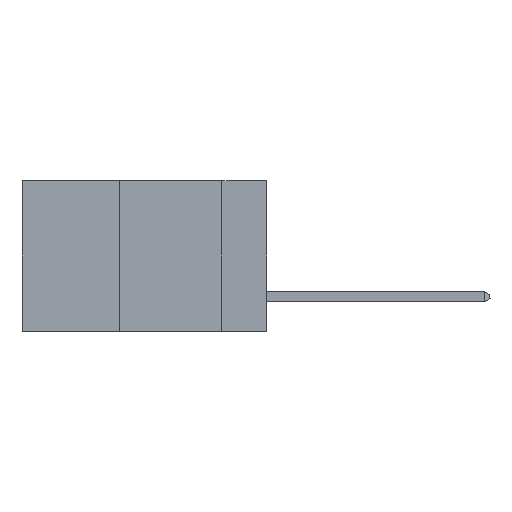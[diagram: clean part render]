
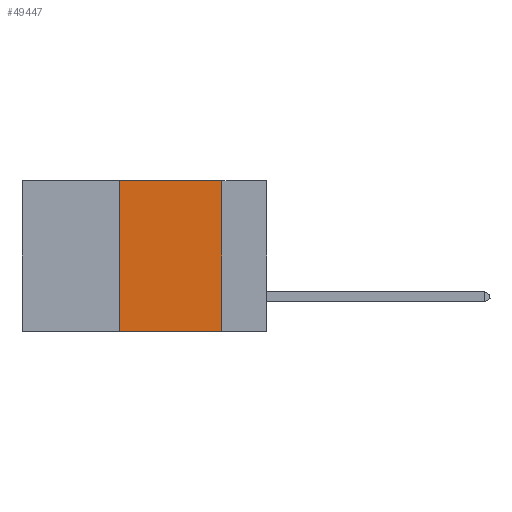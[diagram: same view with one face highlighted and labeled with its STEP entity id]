
A CAD part, left-side view. The second image highlights one B-rep face of the part: STEP entity #49447.
In plain terms, the highlighted planar face has unit normal (-1, 0, 0).
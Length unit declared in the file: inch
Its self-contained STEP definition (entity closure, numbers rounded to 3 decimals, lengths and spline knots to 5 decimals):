
#1496 = CARTESIAN_POINT ( 'NONE',  ( 0., 0.11, 0. ) ) ;
#1722 = ORIENTED_EDGE ( 'NONE', *, *, #30733, .F. ) ;
#4091 = VECTOR ( 'NONE', #8374, 39.37008 ) ;
#4512 = DIRECTION ( 'NONE',  ( 1., 0., 0. ) ) ;
#5875 = CARTESIAN_POINT ( 'NONE',  ( 0., 0.36, 0. ) ) ;
#6215 = EDGE_CURVE ( 'NONE', #12604, #32847, #15452, .T. ) ;
#8374 = DIRECTION ( 'NONE',  ( 0., -1., 0. ) ) ;
#9515 = CARTESIAN_POINT ( 'NONE',  ( 0., 0.6, 0. ) ) ;
#9698 = DIRECTION ( 'NONE',  ( 0., 0., 1. ) ) ;
#11397 = ORIENTED_EDGE ( 'NONE', *, *, #6215, .T. ) ;
#12604 = VERTEX_POINT ( 'NONE', #22365 ) ;
#15452 = LINE ( 'NONE', #35039, #4091 ) ;
#17332 = LINE ( 'NONE', #5875, #37721 ) ;
#17726 = EDGE_CURVE ( 'NONE', #12604, #44195, #17332, .T. ) ;
#18504 = CARTESIAN_POINT ( 'NONE',  ( 0., 0.36, 0. ) ) ;
#18522 = VECTOR ( 'NONE', #24073, 39.37008 ) ;
#20401 = FACE_OUTER_BOUND ( 'NONE', #23271, .T. ) ;
#21495 = EDGE_CURVE ( 'NONE', #44195, #21532, #23572, .T. ) ;
#21532 = VERTEX_POINT ( 'NONE', #1496 ) ;
#22365 = CARTESIAN_POINT ( 'NONE',  ( 0., 0.36, -0.37 ) ) ;
#23271 = EDGE_LOOP ( 'NONE', ( #1722, #43725, #41071, #11397 ) ) ;
#23572 = LINE ( 'NONE', #35117, #24774 ) ;
#24073 = DIRECTION ( 'NONE',  ( 0., 0., -1. ) ) ;
#24774 = VECTOR ( 'NONE', #35286, 39.37008 ) ;
#26397 = CARTESIAN_POINT ( 'NONE',  ( 0., 0.11, -0.37 ) ) ;
#27787 = DIRECTION ( 'NONE',  ( 0., 0., -1. ) ) ;
#30733 = EDGE_CURVE ( 'NONE', #21532, #32847, #38915, .T. ) ;
#32847 = VERTEX_POINT ( 'NONE', #26397 ) ;
#35039 = CARTESIAN_POINT ( 'NONE',  ( 0., 0.6, -0.37 ) ) ;
#35117 = CARTESIAN_POINT ( 'NONE',  ( 0., 0.6, 0. ) ) ;
#35286 = DIRECTION ( 'NONE',  ( 0., -1., 0. ) ) ;
#35463 = CARTESIAN_POINT ( 'NONE',  ( 0., 0.11, 0. ) ) ;
#37721 = VECTOR ( 'NONE', #9698, 39.37008 ) ;
#38566 = AXIS2_PLACEMENT_3D ( 'NONE', #9515, #4512, #27787 ) ;
#38915 = LINE ( 'NONE', #35463, #18522 ) ;
#41071 = ORIENTED_EDGE ( 'NONE', *, *, #17726, .F. ) ;
#43036 = PLANE ( 'NONE',  #38566 ) ;
#43725 = ORIENTED_EDGE ( 'NONE', *, *, #21495, .F. ) ;
#44195 = VERTEX_POINT ( 'NONE', #18504 ) ;
#49447 = ADVANCED_FACE ( 'NONE', ( #20401 ), #43036, .F. ) ;
